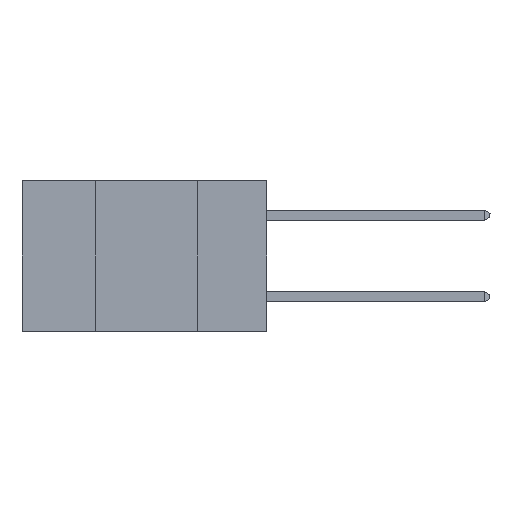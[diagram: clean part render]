
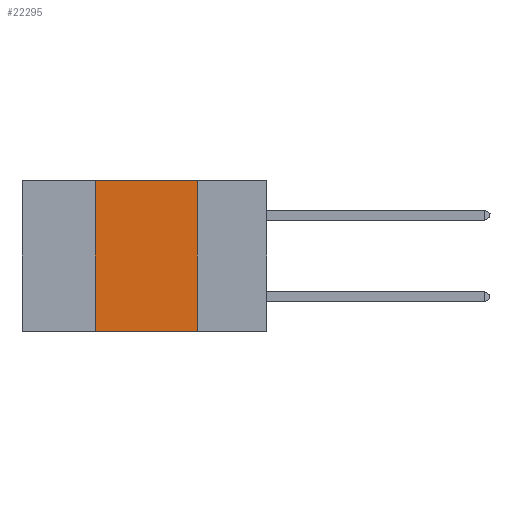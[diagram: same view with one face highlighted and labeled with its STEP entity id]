
A CAD part, left-side view. The second image highlights one B-rep face of the part: STEP entity #22295.
In plain terms, the highlighted planar face has unit normal (-1, 0, 0).
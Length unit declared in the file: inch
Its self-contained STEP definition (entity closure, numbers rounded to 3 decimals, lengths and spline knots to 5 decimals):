
#1318 = VECTOR ( 'NONE', #19602, 39.37008 ) ;
#1355 = VERTEX_POINT ( 'NONE', #3634 ) ;
#3187 = EDGE_CURVE ( 'NONE', #8020, #1355, #33915, .T. ) ;
#3215 = EDGE_CURVE ( 'NONE', #25898, #25959, #12041, .T. ) ;
#3634 = CARTESIAN_POINT ( 'NONE',  ( 0., 0.17, 0. ) ) ;
#4489 = EDGE_LOOP ( 'NONE', ( #21561, #34671, #15035, #30445 ) ) ;
#4828 = LINE ( 'NONE', #10943, #13822 ) ;
#4908 = CARTESIAN_POINT ( 'NONE',  ( 0., 0.6, 0. ) ) ;
#6273 = CARTESIAN_POINT ( 'NONE',  ( 0., 0.17, 0. ) ) ;
#6661 = CARTESIAN_POINT ( 'NONE',  ( 0., 0.6, -0.37 ) ) ;
#7894 = DIRECTION ( 'NONE',  ( 0., 0., 1. ) ) ;
#8020 = VERTEX_POINT ( 'NONE', #33463 ) ;
#10943 = CARTESIAN_POINT ( 'NONE',  ( 0., 0.42, 0. ) ) ;
#12041 = LINE ( 'NONE', #6661, #34000 ) ;
#12991 = DIRECTION ( 'NONE',  ( 1., 0., 0. ) ) ;
#13820 = LINE ( 'NONE', #6273, #19031 ) ;
#13822 = VECTOR ( 'NONE', #7894, 39.37008 ) ;
#15035 = ORIENTED_EDGE ( 'NONE', *, *, #28182, .F. ) ;
#15675 = PLANE ( 'NONE',  #29610 ) ;
#16159 = EDGE_CURVE ( 'NONE', #1355, #25959, #13820, .T. ) ;
#17615 = DIRECTION ( 'NONE',  ( 0., -1., 0. ) ) ;
#18935 = DIRECTION ( 'NONE',  ( 0., 0., -1. ) ) ;
#19031 = VECTOR ( 'NONE', #25100, 39.37008 ) ;
#19602 = DIRECTION ( 'NONE',  ( 0., -1., 0. ) ) ;
#21561 = ORIENTED_EDGE ( 'NONE', *, *, #16159, .F. ) ;
#22295 = ADVANCED_FACE ( 'NONE', ( #29837 ), #15675, .F. ) ;
#22663 = CARTESIAN_POINT ( 'NONE',  ( 0., 0.17, -0.37 ) ) ;
#25100 = DIRECTION ( 'NONE',  ( 0., 0., -1. ) ) ;
#25655 = CARTESIAN_POINT ( 'NONE',  ( 0., 0.6, 0. ) ) ;
#25898 = VERTEX_POINT ( 'NONE', #26968 ) ;
#25959 = VERTEX_POINT ( 'NONE', #22663 ) ;
#26968 = CARTESIAN_POINT ( 'NONE',  ( 0., 0.42, -0.37 ) ) ;
#28182 = EDGE_CURVE ( 'NONE', #25898, #8020, #4828, .T. ) ;
#29610 = AXIS2_PLACEMENT_3D ( 'NONE', #4908, #12991, #18935 ) ;
#29837 = FACE_OUTER_BOUND ( 'NONE', #4489, .T. ) ;
#30445 = ORIENTED_EDGE ( 'NONE', *, *, #3215, .T. ) ;
#33463 = CARTESIAN_POINT ( 'NONE',  ( 0., 0.42, 0. ) ) ;
#33915 = LINE ( 'NONE', #25655, #1318 ) ;
#34000 = VECTOR ( 'NONE', #17615, 39.37008 ) ;
#34671 = ORIENTED_EDGE ( 'NONE', *, *, #3187, .F. ) ;
